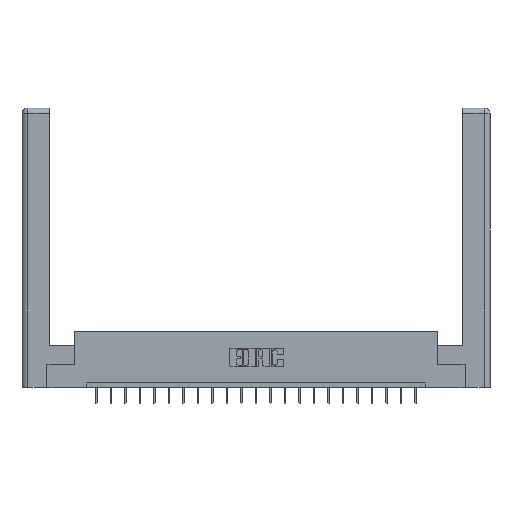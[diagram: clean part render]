
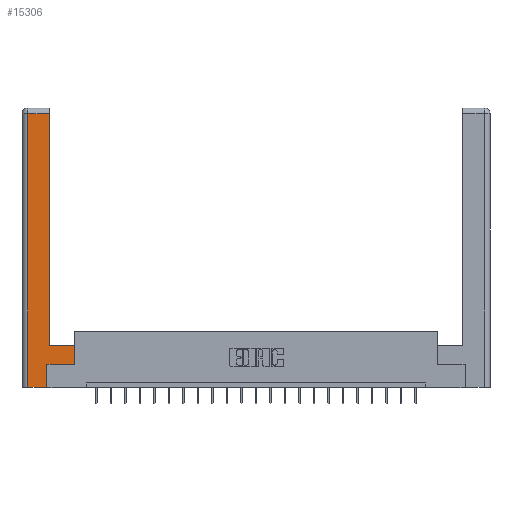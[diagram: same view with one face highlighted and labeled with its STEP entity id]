
A CAD part, top view. The second image highlights one B-rep face of the part: STEP entity #15306.
In plain terms, the highlighted planar face has unit normal (0, 0, 1).
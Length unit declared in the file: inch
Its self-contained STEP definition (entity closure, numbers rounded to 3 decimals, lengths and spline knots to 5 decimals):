
#52 = ORIENTED_EDGE ( 'NONE', *, *, #3249, .T. ) ;
#586 = DIRECTION ( 'NONE',  ( 0., 0., -1. ) ) ;
#717 = ORIENTED_EDGE ( 'NONE', *, *, #21835, .T. ) ;
#728 = CARTESIAN_POINT ( 'NONE',  ( 0.0615, 0., 0. ) ) ;
#854 = CARTESIAN_POINT ( 'NONE',  ( 0.265, 0., 0. ) ) ;
#1108 = VERTEX_POINT ( 'NONE', #19938 ) ;
#1200 = AXIS2_PLACEMENT_3D ( 'NONE', #5574, #586, #5726 ) ;
#1329 = DIRECTION ( 'NONE',  ( 0., 1., 0. ) ) ;
#1402 = CARTESIAN_POINT ( 'NONE',  ( 0.295, 0.45, 0. ) ) ;
#1516 = VECTOR ( 'NONE', #13217, 39.37008 ) ;
#1529 = VECTOR ( 'NONE', #18317, 39.37008 ) ;
#1550 = LINE ( 'NONE', #16310, #21964 ) ;
#2155 = PLANE ( 'NONE',  #1200 ) ;
#2287 = VECTOR ( 'NONE', #13746, 39.37008 ) ;
#2539 = ORIENTED_EDGE ( 'NONE', *, *, #15917, .T. ) ;
#3040 = VERTEX_POINT ( 'NONE', #854 ) ;
#3230 = LINE ( 'NONE', #20133, #12599 ) ;
#3249 = EDGE_CURVE ( 'NONE', #3040, #1108, #4512, .T. ) ;
#3297 = ORIENTED_EDGE ( 'NONE', *, *, #5028, .T. ) ;
#3460 = VECTOR ( 'NONE', #16656, 39.37008 ) ;
#3565 = CARTESIAN_POINT ( 'NONE',  ( 0.0615, 2.94, 0. ) ) ;
#3997 = VERTEX_POINT ( 'NONE', #19461 ) ;
#4512 = LINE ( 'NONE', #11374, #3460 ) ;
#5028 = EDGE_CURVE ( 'NONE', #1108, #3997, #6819, .T. ) ;
#5574 = CARTESIAN_POINT ( 'NONE',  ( 0., 0., 0. ) ) ;
#5726 = DIRECTION ( 'NONE',  ( -1., 0., 0. ) ) ;
#5771 = LINE ( 'NONE', #5921, #1516 ) ;
#5921 = CARTESIAN_POINT ( 'NONE',  ( 0.0615, 2.94, 0. ) ) ;
#6164 = DIRECTION ( 'NONE',  ( 1., 0., 0. ) ) ;
#6413 = VERTEX_POINT ( 'NONE', #3565 ) ;
#6459 = VECTOR ( 'NONE', #19191, 39.37008 ) ;
#6696 = LINE ( 'NONE', #1402, #9386 ) ;
#6819 = LINE ( 'NONE', #11978, #2287 ) ;
#7378 = LINE ( 'NONE', #20339, #1529 ) ;
#7997 = CARTESIAN_POINT ( 'NONE',  ( 0.295, 0.45, 0. ) ) ;
#8337 = VERTEX_POINT ( 'NONE', #7997 ) ;
#9193 = ORIENTED_EDGE ( 'NONE', *, *, #13642, .T. ) ;
#9268 = EDGE_CURVE ( 'NONE', #8337, #18734, #22081, .T. ) ;
#9386 = VECTOR ( 'NONE', #13240, 39.37008 ) ;
#11374 = CARTESIAN_POINT ( 'NONE',  ( 0.265, 0.245, 0. ) ) ;
#11978 = CARTESIAN_POINT ( 'NONE',  ( 0.565, 0.245, 0. ) ) ;
#12599 = VECTOR ( 'NONE', #1329, 39.37008 ) ;
#13217 = DIRECTION ( 'NONE',  ( -1., 0., 0. ) ) ;
#13240 = DIRECTION ( 'NONE',  ( -1., 0., 0. ) ) ;
#13642 = EDGE_CURVE ( 'NONE', #17950, #8337, #6696, .T. ) ;
#13696 = EDGE_CURVE ( 'NONE', #3997, #17950, #3230, .T. ) ;
#13746 = DIRECTION ( 'NONE',  ( 1., 0., 0. ) ) ;
#13950 = CARTESIAN_POINT ( 'NONE',  ( 0.295, 3., 0. ) ) ;
#14430 = ORIENTED_EDGE ( 'NONE', *, *, #20169, .T. ) ;
#15306 = ADVANCED_FACE ( 'NONE', ( #15769 ), #2155, .F. ) ;
#15707 = ORIENTED_EDGE ( 'NONE', *, *, #13696, .T. ) ;
#15769 = FACE_OUTER_BOUND ( 'NONE', #16162, .T. ) ;
#15917 = EDGE_CURVE ( 'NONE', #6413, #16414, #7378, .T. ) ;
#16162 = EDGE_LOOP ( 'NONE', ( #20565, #717, #2539, #14430, #52, #3297, #15707, #9193 ) ) ;
#16310 = CARTESIAN_POINT ( 'NONE',  ( 0.265, 0., 0. ) ) ;
#16414 = VERTEX_POINT ( 'NONE', #728 ) ;
#16656 = DIRECTION ( 'NONE',  ( 0., 1., 0. ) ) ;
#17950 = VERTEX_POINT ( 'NONE', #22028 ) ;
#18317 = DIRECTION ( 'NONE',  ( 0., -1., 0. ) ) ;
#18734 = VERTEX_POINT ( 'NONE', #22267 ) ;
#19191 = DIRECTION ( 'NONE',  ( 0., 1., 0. ) ) ;
#19461 = CARTESIAN_POINT ( 'NONE',  ( 0.565, 0.245, 0. ) ) ;
#19938 = CARTESIAN_POINT ( 'NONE',  ( 0.265, 0.245, 0. ) ) ;
#20133 = CARTESIAN_POINT ( 'NONE',  ( 0.565, 0.45, 0. ) ) ;
#20169 = EDGE_CURVE ( 'NONE', #16414, #3040, #1550, .T. ) ;
#20339 = CARTESIAN_POINT ( 'NONE',  ( 0.0615, 0., 0. ) ) ;
#20565 = ORIENTED_EDGE ( 'NONE', *, *, #9268, .T. ) ;
#21835 = EDGE_CURVE ( 'NONE', #18734, #6413, #5771, .T. ) ;
#21964 = VECTOR ( 'NONE', #6164, 39.37008 ) ;
#22028 = CARTESIAN_POINT ( 'NONE',  ( 0.565, 0.45, 0. ) ) ;
#22081 = LINE ( 'NONE', #13950, #6459 ) ;
#22267 = CARTESIAN_POINT ( 'NONE',  ( 0.295, 2.94, 0. ) ) ;
